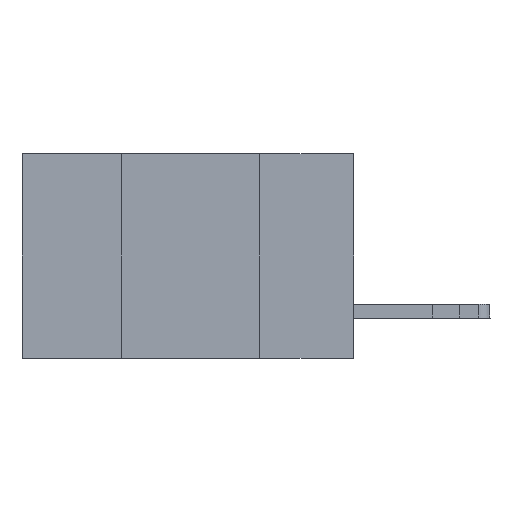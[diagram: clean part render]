
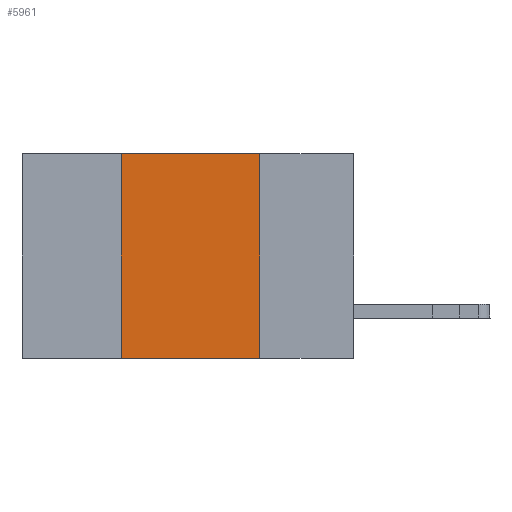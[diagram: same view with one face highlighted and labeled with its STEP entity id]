
A CAD part, left-side view. The second image highlights one B-rep face of the part: STEP entity #5961.
In plain terms, the highlighted planar face has unit normal (-1, 0, 0).
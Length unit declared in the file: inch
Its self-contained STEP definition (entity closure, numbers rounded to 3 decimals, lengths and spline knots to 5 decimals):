
#83 = CARTESIAN_POINT ( 'NONE',  ( 0., 0.42, 0. ) ) ;
#107 = DIRECTION ( 'NONE',  ( 0., 0., -1. ) ) ;
#1326 = ORIENTED_EDGE ( 'NONE', *, *, #6808, .F. ) ;
#1385 = ORIENTED_EDGE ( 'NONE', *, *, #12273, .F. ) ;
#1408 = VERTEX_POINT ( 'NONE', #2068 ) ;
#1951 = EDGE_CURVE ( 'NONE', #1408, #5840, #9788, .T. ) ;
#2068 = CARTESIAN_POINT ( 'NONE',  ( 0., 0.42, -0.37 ) ) ;
#2375 = CARTESIAN_POINT ( 'NONE',  ( 0., 0.42, 0. ) ) ;
#2488 = CARTESIAN_POINT ( 'NONE',  ( 0., 0.17, 0. ) ) ;
#4038 = PLANE ( 'NONE',  #6443 ) ;
#4528 = DIRECTION ( 'NONE',  ( 0., -1., 0. ) ) ;
#4574 = LINE ( 'NONE', #11653, #11270 ) ;
#4989 = EDGE_CURVE ( 'NONE', #1408, #13125, #8897, .T. ) ;
#5135 = VERTEX_POINT ( 'NONE', #2488 ) ;
#5840 = VERTEX_POINT ( 'NONE', #83 ) ;
#5961 = ADVANCED_FACE ( 'NONE', ( #13591 ), #4038, .F. ) ;
#6309 = DIRECTION ( 'NONE',  ( 0., 0., -1. ) ) ;
#6443 = AXIS2_PLACEMENT_3D ( 'NONE', #13899, #12398, #6309 ) ;
#6808 = EDGE_CURVE ( 'NONE', #5840, #5135, #14113, .T. ) ;
#8897 = LINE ( 'NONE', #9928, #16180 ) ;
#9704 = DIRECTION ( 'NONE',  ( 0., -1., 0. ) ) ;
#9788 = LINE ( 'NONE', #2375, #13645 ) ;
#9928 = CARTESIAN_POINT ( 'NONE',  ( 0., 0.6, -0.37 ) ) ;
#10876 = VECTOR ( 'NONE', #4528, 39.37008 ) ;
#11270 = VECTOR ( 'NONE', #107, 39.37008 ) ;
#11364 = CARTESIAN_POINT ( 'NONE',  ( 0., 0.17, -0.37 ) ) ;
#11653 = CARTESIAN_POINT ( 'NONE',  ( 0., 0.17, 0. ) ) ;
#12273 = EDGE_CURVE ( 'NONE', #5135, #13125, #4574, .T. ) ;
#12398 = DIRECTION ( 'NONE',  ( 1., 0., 0. ) ) ;
#12420 = CARTESIAN_POINT ( 'NONE',  ( 0., 0.6, 0. ) ) ;
#13125 = VERTEX_POINT ( 'NONE', #11364 ) ;
#13490 = EDGE_LOOP ( 'NONE', ( #1385, #1326, #16860, #16653 ) ) ;
#13591 = FACE_OUTER_BOUND ( 'NONE', #13490, .T. ) ;
#13645 = VECTOR ( 'NONE', #14167, 39.37008 ) ;
#13899 = CARTESIAN_POINT ( 'NONE',  ( 0., 0.6, 0. ) ) ;
#14113 = LINE ( 'NONE', #12420, #10876 ) ;
#14167 = DIRECTION ( 'NONE',  ( 0., 0., 1. ) ) ;
#16180 = VECTOR ( 'NONE', #9704, 39.37008 ) ;
#16653 = ORIENTED_EDGE ( 'NONE', *, *, #4989, .T. ) ;
#16860 = ORIENTED_EDGE ( 'NONE', *, *, #1951, .F. ) ;
